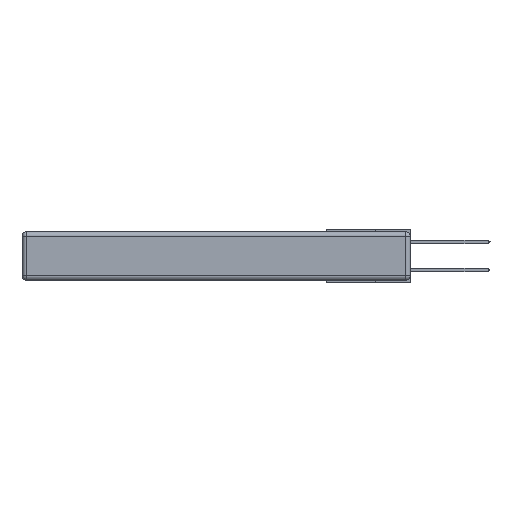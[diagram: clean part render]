
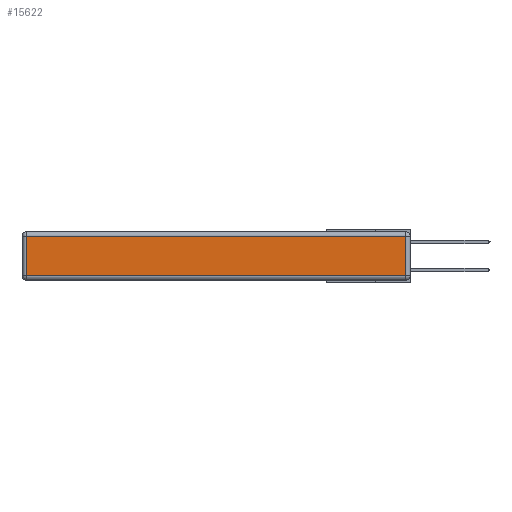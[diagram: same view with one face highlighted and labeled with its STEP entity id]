
A CAD part, left-side view. The second image highlights one B-rep face of the part: STEP entity #15622.
In plain terms, the highlighted planar face has unit normal (-1, 0, 0).
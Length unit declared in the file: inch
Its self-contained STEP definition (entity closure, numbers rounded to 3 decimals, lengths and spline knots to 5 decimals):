
#419 = CARTESIAN_POINT ( 'NONE',  ( 0., 0., -0.343 ) ) ;
#494 = CARTESIAN_POINT ( 'NONE',  ( 0., 0., -0.313 ) ) ;
#628 = PLANE ( 'NONE',  #15287 ) ;
#1142 = CARTESIAN_POINT ( 'NONE',  ( 0., 2.72, -0.313 ) ) ;
#1701 = EDGE_CURVE ( 'NONE', #3387, #17375, #5966, .T. ) ;
#2884 = DIRECTION ( 'NONE',  ( 0., -1., 0. ) ) ;
#3014 = DIRECTION ( 'NONE',  ( 0., 0., 1. ) ) ;
#3387 = VERTEX_POINT ( 'NONE', #8840 ) ;
#4597 = CARTESIAN_POINT ( 'NONE',  ( 0., 2.72, -0.343 ) ) ;
#5966 = LINE ( 'NONE', #27591, #25784 ) ;
#6356 = ORIENTED_EDGE ( 'NONE', *, *, #12671, .T. ) ;
#7130 = ORIENTED_EDGE ( 'NONE', *, *, #22973, .T. ) ;
#7901 = DIRECTION ( 'NONE',  ( 0., 1., 0. ) ) ;
#8295 = VERTEX_POINT ( 'NONE', #1142 ) ;
#8428 = CARTESIAN_POINT ( 'NONE',  ( 0., 2.72, -0.03 ) ) ;
#8443 = DIRECTION ( 'NONE',  ( 0., 0., 1. ) ) ;
#8840 = CARTESIAN_POINT ( 'NONE',  ( 0., 0.03, -0.03 ) ) ;
#12671 = EDGE_CURVE ( 'NONE', #8295, #19547, #14105, .T. ) ;
#12683 = VECTOR ( 'NONE', #29273, 39.37008 ) ;
#14105 = LINE ( 'NONE', #494, #20335 ) ;
#15168 = DIRECTION ( 'NONE',  ( -1., 0., 0. ) ) ;
#15287 = AXIS2_PLACEMENT_3D ( 'NONE', #419, #15168, #3014 ) ;
#15513 = FACE_OUTER_BOUND ( 'NONE', #16711, .T. ) ;
#15622 = ADVANCED_FACE ( 'NONE', ( #15513 ), #628, .T. ) ;
#16711 = EDGE_LOOP ( 'NONE', ( #6356, #7130, #31869, #22911 ) ) ;
#16767 = EDGE_CURVE ( 'NONE', #17375, #8295, #25923, .T. ) ;
#17375 = VERTEX_POINT ( 'NONE', #8428 ) ;
#19547 = VERTEX_POINT ( 'NONE', #27725 ) ;
#20335 = VECTOR ( 'NONE', #2884, 39.37008 ) ;
#22911 = ORIENTED_EDGE ( 'NONE', *, *, #16767, .T. ) ;
#22973 = EDGE_CURVE ( 'NONE', #19547, #3387, #24431, .T. ) ;
#24431 = LINE ( 'NONE', #30700, #27129 ) ;
#25784 = VECTOR ( 'NONE', #7901, 39.37008 ) ;
#25923 = LINE ( 'NONE', #4597, #12683 ) ;
#27129 = VECTOR ( 'NONE', #8443, 39.37008 ) ;
#27591 = CARTESIAN_POINT ( 'NONE',  ( 0., 2.75, -0.03 ) ) ;
#27725 = CARTESIAN_POINT ( 'NONE',  ( 0., 0.03, -0.313 ) ) ;
#29273 = DIRECTION ( 'NONE',  ( 0., 0., -1. ) ) ;
#30700 = CARTESIAN_POINT ( 'NONE',  ( 0., 0.03, -0.343 ) ) ;
#31869 = ORIENTED_EDGE ( 'NONE', *, *, #1701, .T. ) ;
